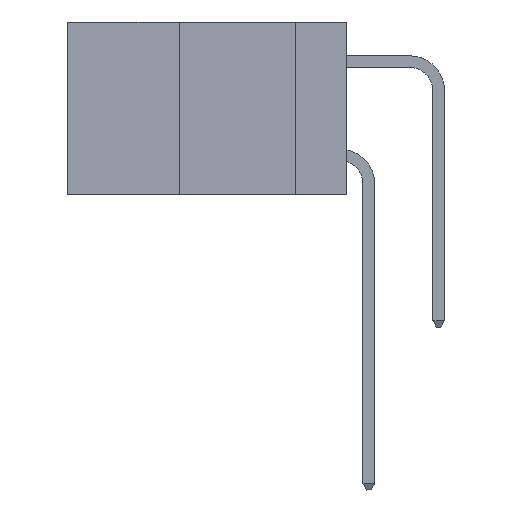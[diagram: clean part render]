
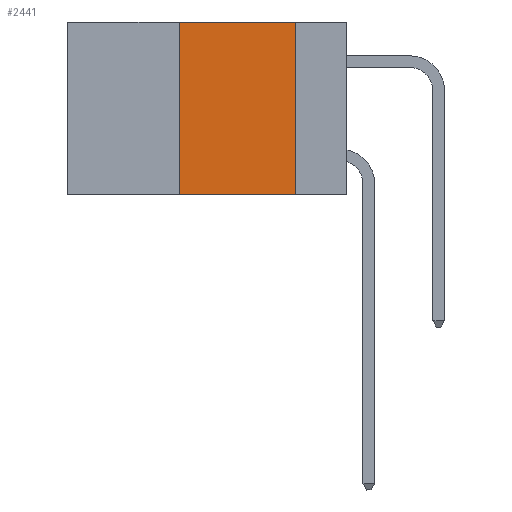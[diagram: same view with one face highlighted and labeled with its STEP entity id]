
A CAD part, left-side view. The second image highlights one B-rep face of the part: STEP entity #2441.
In plain terms, the highlighted planar face has unit normal (-1, 0, 0).
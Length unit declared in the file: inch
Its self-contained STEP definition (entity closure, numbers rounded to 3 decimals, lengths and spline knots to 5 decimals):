
#82 = LINE ( 'NONE', #8162, #24843 ) ;
#282 = CARTESIAN_POINT ( 'NONE',  ( 0., 0.6, 0. ) ) ;
#2362 = VERTEX_POINT ( 'NONE', #9278 ) ;
#2441 = ADVANCED_FACE ( 'NONE', ( #18099 ), #16133, .F. ) ;
#2716 = VECTOR ( 'NONE', #19881, 39.37008 ) ;
#3590 = DIRECTION ( 'NONE',  ( 1., 0., 0. ) ) ;
#4679 = ORIENTED_EDGE ( 'NONE', *, *, #17966, .F. ) ;
#6156 = VERTEX_POINT ( 'NONE', #22249 ) ;
#7064 = CARTESIAN_POINT ( 'NONE',  ( 0., 0.36, 0. ) ) ;
#8162 = CARTESIAN_POINT ( 'NONE',  ( 0., 0.6, 0. ) ) ;
#8446 = CARTESIAN_POINT ( 'NONE',  ( 0., 0.11, 0. ) ) ;
#9278 = CARTESIAN_POINT ( 'NONE',  ( 0., 0.36, -0.37 ) ) ;
#9716 = VECTOR ( 'NONE', #22893, 39.37008 ) ;
#13240 = VECTOR ( 'NONE', #15107, 39.37008 ) ;
#13720 = CARTESIAN_POINT ( 'NONE',  ( 0., 0.6, -0.37 ) ) ;
#14719 = LINE ( 'NONE', #20756, #9716 ) ;
#15107 = DIRECTION ( 'NONE',  ( 0., 0., 1. ) ) ;
#15478 = VERTEX_POINT ( 'NONE', #8446 ) ;
#15606 = DIRECTION ( 'NONE',  ( 0., 0., -1. ) ) ;
#16133 = PLANE ( 'NONE',  #22346 ) ;
#16227 = DIRECTION ( 'NONE',  ( 0., -1., 0. ) ) ;
#17070 = EDGE_LOOP ( 'NONE', ( #4679, #23716, #19961, #21436 ) ) ;
#17311 = EDGE_CURVE ( 'NONE', #20334, #15478, #82, .T. ) ;
#17966 = EDGE_CURVE ( 'NONE', #15478, #6156, #14719, .T. ) ;
#18099 = FACE_OUTER_BOUND ( 'NONE', #17070, .T. ) ;
#19881 = DIRECTION ( 'NONE',  ( 0., -1., 0. ) ) ;
#19961 = ORIENTED_EDGE ( 'NONE', *, *, #22103, .F. ) ;
#20334 = VERTEX_POINT ( 'NONE', #25282 ) ;
#20756 = CARTESIAN_POINT ( 'NONE',  ( 0., 0.11, 0. ) ) ;
#21436 = ORIENTED_EDGE ( 'NONE', *, *, #24657, .T. ) ;
#22103 = EDGE_CURVE ( 'NONE', #2362, #20334, #23024, .T. ) ;
#22249 = CARTESIAN_POINT ( 'NONE',  ( 0., 0.11, -0.37 ) ) ;
#22346 = AXIS2_PLACEMENT_3D ( 'NONE', #282, #3590, #15606 ) ;
#22893 = DIRECTION ( 'NONE',  ( 0., 0., -1. ) ) ;
#23024 = LINE ( 'NONE', #7064, #13240 ) ;
#23716 = ORIENTED_EDGE ( 'NONE', *, *, #17311, .F. ) ;
#23744 = LINE ( 'NONE', #13720, #2716 ) ;
#24657 = EDGE_CURVE ( 'NONE', #2362, #6156, #23744, .T. ) ;
#24843 = VECTOR ( 'NONE', #16227, 39.37008 ) ;
#25282 = CARTESIAN_POINT ( 'NONE',  ( 0., 0.36, 0. ) ) ;
